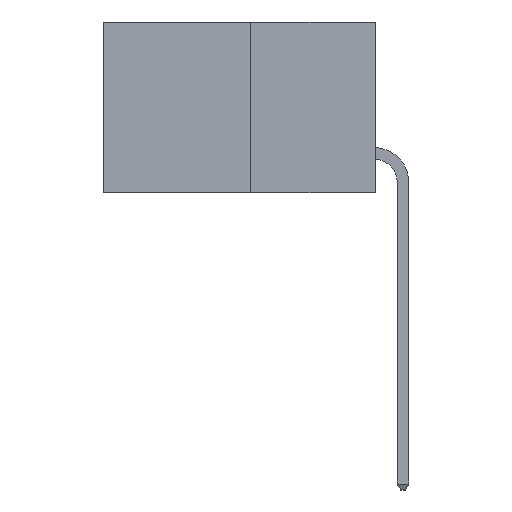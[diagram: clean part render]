
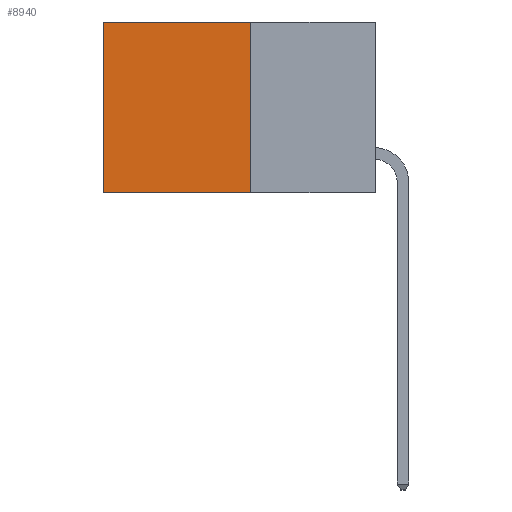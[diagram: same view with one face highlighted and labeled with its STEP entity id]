
A CAD part, left-side view. The second image highlights one B-rep face of the part: STEP entity #8940.
In plain terms, the highlighted planar face has unit normal (-1, 0, 0).
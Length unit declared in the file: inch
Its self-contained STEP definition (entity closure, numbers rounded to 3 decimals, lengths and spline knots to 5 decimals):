
#13 = ORIENTED_EDGE ( 'NONE', *, *, #6044, .F. ) ;
#66 = DIRECTION ( 'NONE',  ( 0., 0., -1. ) ) ;
#83 = AXIS2_PLACEMENT_3D ( 'NONE', #4307, #9761, #5113 ) ;
#471 = CARTESIAN_POINT ( 'NONE',  ( 0.277, 0.59, 0. ) ) ;
#694 = ORIENTED_EDGE ( 'NONE', *, *, #8939, .T. ) ;
#886 = CARTESIAN_POINT ( 'NONE',  ( 0.277, 0.27, 0. ) ) ;
#956 = VECTOR ( 'NONE', #3487, 39.37008 ) ;
#1519 = EDGE_CURVE ( 'NONE', #4613, #8845, #9055, .T. ) ;
#1764 = PLANE ( 'NONE',  #83 ) ;
#2163 = VERTEX_POINT ( 'NONE', #471 ) ;
#2398 = LINE ( 'NONE', #4549, #8506 ) ;
#3253 = FACE_OUTER_BOUND ( 'NONE', #5624, .T. ) ;
#3487 = DIRECTION ( 'NONE',  ( 0., 1., 0. ) ) ;
#4165 = ORIENTED_EDGE ( 'NONE', *, *, #7681, .T. ) ;
#4307 = CARTESIAN_POINT ( 'NONE',  ( 0.277, 0.27, -0.37 ) ) ;
#4476 = CARTESIAN_POINT ( 'NONE',  ( 0.277, 0.27, -0.37 ) ) ;
#4549 = CARTESIAN_POINT ( 'NONE',  ( 0.277, 0.27, -0.37 ) ) ;
#4613 = VERTEX_POINT ( 'NONE', #4476 ) ;
#4913 = VECTOR ( 'NONE', #9670, 39.37008 ) ;
#5055 = ORIENTED_EDGE ( 'NONE', *, *, #1519, .F. ) ;
#5113 = DIRECTION ( 'NONE',  ( 0., 0., -1. ) ) ;
#5190 = VECTOR ( 'NONE', #66, 39.37008 ) ;
#5444 = LINE ( 'NONE', #8245, #5190 ) ;
#5624 = EDGE_LOOP ( 'NONE', ( #4165, #5055, #13, #694 ) ) ;
#5981 = VERTEX_POINT ( 'NONE', #6032 ) ;
#6032 = CARTESIAN_POINT ( 'NONE',  ( 0.277, 0.27, 0. ) ) ;
#6044 = EDGE_CURVE ( 'NONE', #5981, #4613, #2398, .T. ) ;
#6149 = CARTESIAN_POINT ( 'NONE',  ( 0.277, 0.27, -0.37 ) ) ;
#7681 = EDGE_CURVE ( 'NONE', #2163, #8845, #5444, .T. ) ;
#8245 = CARTESIAN_POINT ( 'NONE',  ( 0.277, 0.59, -0.37 ) ) ;
#8506 = VECTOR ( 'NONE', #9234, 39.37008 ) ;
#8845 = VERTEX_POINT ( 'NONE', #8914 ) ;
#8914 = CARTESIAN_POINT ( 'NONE',  ( 0.277, 0.59, -0.37 ) ) ;
#8939 = EDGE_CURVE ( 'NONE', #5981, #2163, #9538, .T. ) ;
#8940 = ADVANCED_FACE ( 'NONE', ( #3253 ), #1764, .F. ) ;
#9055 = LINE ( 'NONE', #6149, #4913 ) ;
#9234 = DIRECTION ( 'NONE',  ( 0., 0., -1. ) ) ;
#9538 = LINE ( 'NONE', #886, #956 ) ;
#9670 = DIRECTION ( 'NONE',  ( 0., 1., 0. ) ) ;
#9761 = DIRECTION ( 'NONE',  ( 1., 0., 0. ) ) ;
